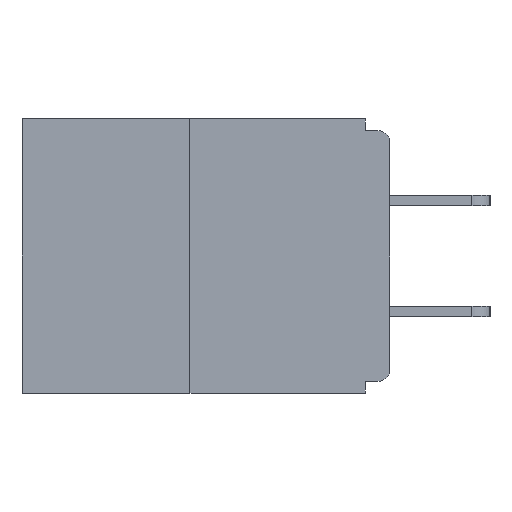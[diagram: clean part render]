
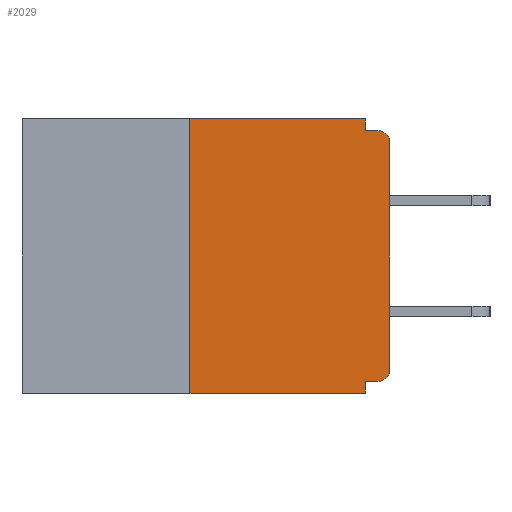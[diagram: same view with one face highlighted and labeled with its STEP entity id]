
A CAD part, left-side view. The second image highlights one B-rep face of the part: STEP entity #2029.
In plain terms, the highlighted planar face has unit normal (-1, 0, 0).
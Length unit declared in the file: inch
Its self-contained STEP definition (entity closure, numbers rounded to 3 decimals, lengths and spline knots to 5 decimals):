
#262 = CARTESIAN_POINT ( 'NONE',  ( 0., 0.015, -0.015 ) ) ;
#1417 = CARTESIAN_POINT ( 'NONE',  ( 0., 0.25, -0.343 ) ) ;
#1466 = DIRECTION ( 'NONE',  ( 0., -1., 0. ) ) ;
#1815 = DIRECTION ( 'NONE',  ( 0., -1., 0. ) ) ;
#2029 = ADVANCED_FACE ( 'NONE', ( #7828 ), #20917, .F. ) ;
#2584 = EDGE_CURVE ( 'NONE', #6352, #20782, #19155, .T. ) ;
#3112 = LINE ( 'NONE', #6968, #21240 ) ;
#3331 = CARTESIAN_POINT ( 'NONE',  ( 0., 0.015, -0.328 ) ) ;
#3697 = EDGE_CURVE ( 'NONE', #14174, #15501, #22071, .T. ) ;
#3734 = DIRECTION ( 'NONE',  ( 1., 0., 0. ) ) ;
#4798 = DIRECTION ( 'NONE',  ( 0., 0., -1. ) ) ;
#4898 = ORIENTED_EDGE ( 'NONE', *, *, #16269, .T. ) ;
#5022 = ORIENTED_EDGE ( 'NONE', *, *, #11304, .T. ) ;
#5495 = LINE ( 'NONE', #14760, #18082 ) ;
#5897 = CARTESIAN_POINT ( 'NONE',  ( 0., 0., -0.313 ) ) ;
#6230 = CARTESIAN_POINT ( 'NONE',  ( 0., 0.015, -0.03 ) ) ;
#6352 = VERTEX_POINT ( 'NONE', #1417 ) ;
#6571 = VERTEX_POINT ( 'NONE', #14458 ) ;
#6968 = CARTESIAN_POINT ( 'NONE',  ( 0., 0., -0.328 ) ) ;
#7139 = VERTEX_POINT ( 'NONE', #3331 ) ;
#7215 = EDGE_LOOP ( 'NONE', ( #22714, #9792, #18390, #14740, #10526, #4898, #11313, #5022, #21157, #12233 ) ) ;
#7415 = CARTESIAN_POINT ( 'NONE',  ( 0., 0.031, -0.015 ) ) ;
#7828 = FACE_OUTER_BOUND ( 'NONE', #7215, .T. ) ;
#7950 = DIRECTION ( 'NONE',  ( 0., 0., -1. ) ) ;
#8019 = DIRECTION ( 'NONE',  ( -1., 0., 0. ) ) ;
#8183 = DIRECTION ( 'NONE',  ( 0., 0., 1. ) ) ;
#8403 = VECTOR ( 'NONE', #7950, 39.37008 ) ;
#8824 = CARTESIAN_POINT ( 'NONE',  ( 0., 0.031, 0. ) ) ;
#8931 = AXIS2_PLACEMENT_3D ( 'NONE', #21367, #9831, #21252 ) ;
#9008 = DIRECTION ( 'NONE',  ( 0., 1., 0. ) ) ;
#9053 = VERTEX_POINT ( 'NONE', #5897 ) ;
#9440 = CARTESIAN_POINT ( 'NONE',  ( 0., 0., -0.03 ) ) ;
#9591 = CARTESIAN_POINT ( 'NONE',  ( 0., 0.25, 0. ) ) ;
#9689 = LINE ( 'NONE', #20984, #24218 ) ;
#9792 = ORIENTED_EDGE ( 'NONE', *, *, #2584, .F. ) ;
#9831 = DIRECTION ( 'NONE',  ( -1., 0., 0. ) ) ;
#10135 = VECTOR ( 'NONE', #1466, 39.37008 ) ;
#10526 = ORIENTED_EDGE ( 'NONE', *, *, #21656, .F. ) ;
#11181 = AXIS2_PLACEMENT_3D ( 'NONE', #6230, #8019, #19595 ) ;
#11304 = EDGE_CURVE ( 'NONE', #16529, #15501, #15538, .T. ) ;
#11313 = ORIENTED_EDGE ( 'NONE', *, *, #21981, .T. ) ;
#12201 = EDGE_CURVE ( 'NONE', #19098, #6571, #17533, .T. ) ;
#12233 = ORIENTED_EDGE ( 'NONE', *, *, #22808, .F. ) ;
#12322 = VECTOR ( 'NONE', #8183, 39.37008 ) ;
#12613 = CARTESIAN_POINT ( 'NONE',  ( 0., 0., -0.015 ) ) ;
#13050 = DIRECTION ( 'NONE',  ( 0., 0., 1. ) ) ;
#13307 = CIRCLE ( 'NONE', #8931, 0.015 ) ;
#13807 = CARTESIAN_POINT ( 'NONE',  ( 0., 0.46, 0. ) ) ;
#14050 = CARTESIAN_POINT ( 'NONE',  ( 0., 0.031, -0.343 ) ) ;
#14174 = VERTEX_POINT ( 'NONE', #7415 ) ;
#14458 = CARTESIAN_POINT ( 'NONE',  ( 0., 0.031, -0.343 ) ) ;
#14740 = ORIENTED_EDGE ( 'NONE', *, *, #12201, .F. ) ;
#14760 = CARTESIAN_POINT ( 'NONE',  ( 0., 0., 0. ) ) ;
#14993 = CARTESIAN_POINT ( 'NONE',  ( 0., 0.031, -0.328 ) ) ;
#15501 = VERTEX_POINT ( 'NONE', #262 ) ;
#15538 = CIRCLE ( 'NONE', #11181, 0.015 ) ;
#16269 = EDGE_CURVE ( 'NONE', #7139, #9053, #13307, .T. ) ;
#16527 = VECTOR ( 'NONE', #4798, 39.37008 ) ;
#16529 = VERTEX_POINT ( 'NONE', #9440 ) ;
#17533 = LINE ( 'NONE', #14050, #8403 ) ;
#18082 = VECTOR ( 'NONE', #13050, 39.37008 ) ;
#18390 = ORIENTED_EDGE ( 'NONE', *, *, #21475, .T. ) ;
#18545 = CARTESIAN_POINT ( 'NONE',  ( 0., 0.46, -0.343 ) ) ;
#19098 = VERTEX_POINT ( 'NONE', #14993 ) ;
#19155 = LINE ( 'NONE', #9591, #12322 ) ;
#19595 = DIRECTION ( 'NONE',  ( 0., 0., -1. ) ) ;
#19796 = CARTESIAN_POINT ( 'NONE',  ( 0., 0.25, 0. ) ) ;
#20137 = VERTEX_POINT ( 'NONE', #22120 ) ;
#20782 = VERTEX_POINT ( 'NONE', #19796 ) ;
#20813 = VECTOR ( 'NONE', #21678, 39.37008 ) ;
#20917 = PLANE ( 'NONE',  #23442 ) ;
#20984 = CARTESIAN_POINT ( 'NONE',  ( 0., 0.46, 0. ) ) ;
#21157 = ORIENTED_EDGE ( 'NONE', *, *, #3697, .F. ) ;
#21240 = VECTOR ( 'NONE', #9008, 39.37008 ) ;
#21252 = DIRECTION ( 'NONE',  ( 0., 0., -1. ) ) ;
#21367 = CARTESIAN_POINT ( 'NONE',  ( 0., 0.015, -0.313 ) ) ;
#21475 = EDGE_CURVE ( 'NONE', #6352, #6571, #22278, .T. ) ;
#21656 = EDGE_CURVE ( 'NONE', #7139, #19098, #3112, .T. ) ;
#21678 = DIRECTION ( 'NONE',  ( 0., -1., 0. ) ) ;
#21981 = EDGE_CURVE ( 'NONE', #9053, #16529, #5495, .T. ) ;
#22071 = LINE ( 'NONE', #12613, #20813 ) ;
#22120 = CARTESIAN_POINT ( 'NONE',  ( 0., 0.031, 0. ) ) ;
#22278 = LINE ( 'NONE', #18545, #10135 ) ;
#22714 = ORIENTED_EDGE ( 'NONE', *, *, #24235, .F. ) ;
#22808 = EDGE_CURVE ( 'NONE', #20137, #14174, #24254, .T. ) ;
#23030 = DIRECTION ( 'NONE',  ( 0., 0., -1. ) ) ;
#23442 = AXIS2_PLACEMENT_3D ( 'NONE', #13807, #3734, #23030 ) ;
#24218 = VECTOR ( 'NONE', #1815, 39.37008 ) ;
#24235 = EDGE_CURVE ( 'NONE', #20782, #20137, #9689, .T. ) ;
#24254 = LINE ( 'NONE', #8824, #16527 ) ;
